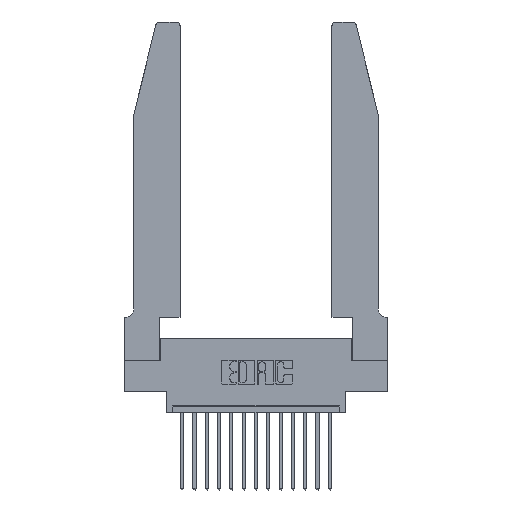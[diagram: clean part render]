
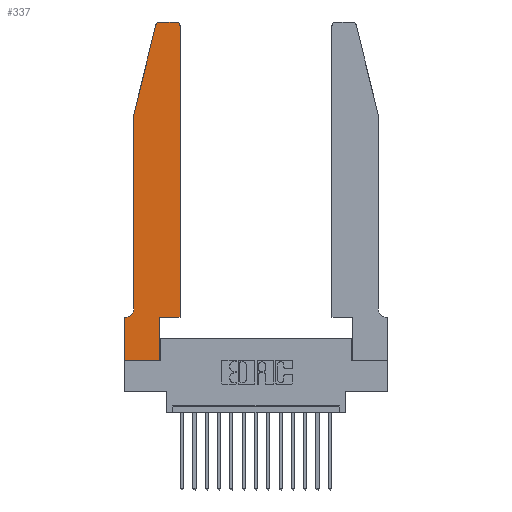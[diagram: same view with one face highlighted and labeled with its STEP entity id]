
A CAD part, top view. The second image highlights one B-rep face of the part: STEP entity #337.
In plain terms, the highlighted planar face has unit normal (0, 0, 1).
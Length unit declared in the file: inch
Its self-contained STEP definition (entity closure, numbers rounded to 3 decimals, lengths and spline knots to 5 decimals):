
#79 = DIRECTION ( 'NONE',  ( -1., 0., 0. ) ) ;
#208 = CARTESIAN_POINT ( 'NONE',  ( 0.2605, 2.75, 0.37 ) ) ;
#337 = ADVANCED_FACE ( 'NONE', ( #7506 ), #13636, .T. ) ;
#688 = CARTESIAN_POINT ( 'NONE',  ( 0.0755, 2., 0.37 ) ) ;
#853 = DIRECTION ( 'NONE',  ( 1., 0., 0. ) ) ;
#1028 = VERTEX_POINT ( 'NONE', #4539 ) ;
#1416 = LINE ( 'NONE', #8061, #12416 ) ;
#2205 = VECTOR ( 'NONE', #8676, 39.37008 ) ;
#2355 = VERTEX_POINT ( 'NONE', #15347 ) ;
#2431 = CIRCLE ( 'NONE', #18123, 0.03 ) ;
#2514 = ORIENTED_EDGE ( 'NONE', *, *, #16900, .T. ) ;
#2862 = VERTEX_POINT ( 'NONE', #15883 ) ;
#3105 = DIRECTION ( 'NONE',  ( 1., 0., 0. ) ) ;
#3220 = DIRECTION ( 'NONE',  ( 1., 0., 0. ) ) ;
#3275 = EDGE_LOOP ( 'NONE', ( #14840, #11677, #5353, #2514, #17677, #6969, #4607, #13292, #12855, #6012, #5278, #12899 ) ) ;
#3391 = CARTESIAN_POINT ( 'NONE',  ( 0., 0., 0.37 ) ) ;
#3401 = DIRECTION ( 'NONE',  ( 0., 1., 0. ) ) ;
#3635 = CARTESIAN_POINT ( 'NONE',  ( 0.4205, 2.72, 0.37 ) ) ;
#3996 = VECTOR ( 'NONE', #79, 39.37008 ) ;
#4057 = LINE ( 'NONE', #6527, #6505 ) ;
#4083 = VECTOR ( 'NONE', #3401, 39.37008 ) ;
#4191 = CARTESIAN_POINT ( 'NONE',  ( 0.0755, 0.42, 0.37 ) ) ;
#4349 = EDGE_CURVE ( 'NONE', #11443, #17301, #9056, .T. ) ;
#4381 = VERTEX_POINT ( 'NONE', #688 ) ;
#4474 = VERTEX_POINT ( 'NONE', #13722 ) ;
#4539 = CARTESIAN_POINT ( 'NONE',  ( 0.284, 2.75, 0.37 ) ) ;
#4607 = ORIENTED_EDGE ( 'NONE', *, *, #6400, .T. ) ;
#5106 = DIRECTION ( 'NONE',  ( 0., 1., 0. ) ) ;
#5153 = CARTESIAN_POINT ( 'NONE',  ( 0., 0.35, 0.37 ) ) ;
#5199 = DIRECTION ( 'NONE',  ( 1., 0., 0. ) ) ;
#5278 = ORIENTED_EDGE ( 'NONE', *, *, #11276, .T. ) ;
#5353 = ORIENTED_EDGE ( 'NONE', *, *, #8972, .T. ) ;
#5357 = CARTESIAN_POINT ( 'NONE',  ( 0.0055, 0.35, 0.37 ) ) ;
#6012 = ORIENTED_EDGE ( 'NONE', *, *, #16632, .T. ) ;
#6145 = VECTOR ( 'NONE', #5106, 39.37008 ) ;
#6328 = AXIS2_PLACEMENT_3D ( 'NONE', #9279, #12264, #12209 ) ;
#6381 = DIRECTION ( 'NONE',  ( -1., 0., 0. ) ) ;
#6400 = EDGE_CURVE ( 'NONE', #9644, #2355, #9851, .T. ) ;
#6505 = VECTOR ( 'NONE', #5199, 39.37008 ) ;
#6527 = CARTESIAN_POINT ( 'NONE',  ( 0.4505, 0.35, 0.37 ) ) ;
#6969 = ORIENTED_EDGE ( 'NONE', *, *, #13978, .T. ) ;
#7050 = DIRECTION ( 'NONE',  ( 0., 0., 1. ) ) ;
#7076 = VERTEX_POINT ( 'NONE', #16909 ) ;
#7444 = CIRCLE ( 'NONE', #6328, 0.07 ) ;
#7506 = FACE_OUTER_BOUND ( 'NONE', #3275, .T. ) ;
#7557 = CIRCLE ( 'NONE', #8092, 0.03 ) ;
#8009 = CARTESIAN_POINT ( 'NONE',  ( 0.284, 2.72, 0.37 ) ) ;
#8039 = EDGE_CURVE ( 'NONE', #17333, #7076, #7557, .T. ) ;
#8061 = CARTESIAN_POINT ( 'NONE',  ( 0.0755, 2., 0.37 ) ) ;
#8092 = AXIS2_PLACEMENT_3D ( 'NONE', #3635, #15091, #10794 ) ;
#8258 = AXIS2_PLACEMENT_3D ( 'NONE', #10815, #7050, #3220 ) ;
#8676 = DIRECTION ( 'NONE',  ( 0., -1., 0. ) ) ;
#8720 = CARTESIAN_POINT ( 'NONE',  ( 0.0755, 0.35, 0.37 ) ) ;
#8844 = CARTESIAN_POINT ( 'NONE',  ( 0., 0., 0.37 ) ) ;
#8972 = EDGE_CURVE ( 'NONE', #2862, #4381, #1416, .T. ) ;
#9056 = LINE ( 'NONE', #16421, #4083 ) ;
#9231 = LINE ( 'NONE', #15938, #2205 ) ;
#9279 = CARTESIAN_POINT ( 'NONE',  ( 0.0055, 0.42, 0.37 ) ) ;
#9474 = DIRECTION ( 'NONE',  ( 0., 0., 1. ) ) ;
#9644 = VERTEX_POINT ( 'NONE', #5153 ) ;
#9851 = LINE ( 'NONE', #3391, #14978 ) ;
#9920 = VECTOR ( 'NONE', #3105, 39.37008 ) ;
#10636 = CARTESIAN_POINT ( 'NONE',  ( 0.4505, 0.35, 0.37 ) ) ;
#10794 = DIRECTION ( 'NONE',  ( 1., 0., 0. ) ) ;
#10815 = CARTESIAN_POINT ( 'NONE',  ( 0., 0.35, 0.37 ) ) ;
#10932 = VERTEX_POINT ( 'NONE', #4191 ) ;
#11276 = EDGE_CURVE ( 'NONE', #4474, #17333, #13314, .T. ) ;
#11443 = VERTEX_POINT ( 'NONE', #12162 ) ;
#11677 = ORIENTED_EDGE ( 'NONE', *, *, #13505, .T. ) ;
#12162 = CARTESIAN_POINT ( 'NONE',  ( 0.2865, 0., 0.37 ) ) ;
#12209 = DIRECTION ( 'NONE',  ( -1., 0., 0. ) ) ;
#12264 = DIRECTION ( 'NONE',  ( 0., 0., -1. ) ) ;
#12416 = VECTOR ( 'NONE', #18366, 39.37008 ) ;
#12461 = EDGE_CURVE ( 'NONE', #2355, #11443, #16626, .T. ) ;
#12610 = EDGE_CURVE ( 'NONE', #10932, #14336, #7444, .T. ) ;
#12855 = ORIENTED_EDGE ( 'NONE', *, *, #4349, .T. ) ;
#12899 = ORIENTED_EDGE ( 'NONE', *, *, #8039, .T. ) ;
#13292 = ORIENTED_EDGE ( 'NONE', *, *, #12461, .T. ) ;
#13314 = LINE ( 'NONE', #10636, #6145 ) ;
#13414 = DIRECTION ( 'NONE',  ( 0., -1., 0. ) ) ;
#13505 = EDGE_CURVE ( 'NONE', #1028, #2862, #2431, .T. ) ;
#13636 = PLANE ( 'NONE',  #8258 ) ;
#13722 = CARTESIAN_POINT ( 'NONE',  ( 0.4505, 0.35, 0.37 ) ) ;
#13978 = EDGE_CURVE ( 'NONE', #14336, #9644, #14338, .T. ) ;
#14132 = CARTESIAN_POINT ( 'NONE',  ( 0.4505, 2.72, 0.37 ) ) ;
#14336 = VERTEX_POINT ( 'NONE', #5357 ) ;
#14338 = LINE ( 'NONE', #8720, #17047 ) ;
#14543 = LINE ( 'NONE', #208, #3996 ) ;
#14840 = ORIENTED_EDGE ( 'NONE', *, *, #18117, .T. ) ;
#14978 = VECTOR ( 'NONE', #13414, 39.37008 ) ;
#15091 = DIRECTION ( 'NONE',  ( 0., 0., 1. ) ) ;
#15347 = CARTESIAN_POINT ( 'NONE',  ( 0., 0., 0.37 ) ) ;
#15883 = CARTESIAN_POINT ( 'NONE',  ( 0.25487, 2.72718, 0.37 ) ) ;
#15938 = CARTESIAN_POINT ( 'NONE',  ( 0.0755, 2., 0.37 ) ) ;
#16421 = CARTESIAN_POINT ( 'NONE',  ( 0.2865, 0.35, 0.37 ) ) ;
#16626 = LINE ( 'NONE', #8844, #9920 ) ;
#16632 = EDGE_CURVE ( 'NONE', #17301, #4474, #4057, .T. ) ;
#16767 = CARTESIAN_POINT ( 'NONE',  ( 0.2865, 0.35, 0.37 ) ) ;
#16900 = EDGE_CURVE ( 'NONE', #4381, #10932, #9231, .T. ) ;
#16909 = CARTESIAN_POINT ( 'NONE',  ( 0.4205, 2.75, 0.37 ) ) ;
#17047 = VECTOR ( 'NONE', #6381, 39.37008 ) ;
#17301 = VERTEX_POINT ( 'NONE', #16767 ) ;
#17333 = VERTEX_POINT ( 'NONE', #14132 ) ;
#17677 = ORIENTED_EDGE ( 'NONE', *, *, #12610, .T. ) ;
#18117 = EDGE_CURVE ( 'NONE', #7076, #1028, #14543, .T. ) ;
#18123 = AXIS2_PLACEMENT_3D ( 'NONE', #8009, #9474, #853 ) ;
#18366 = DIRECTION ( 'NONE',  ( -0.239, -0.971, 0. ) ) ;
